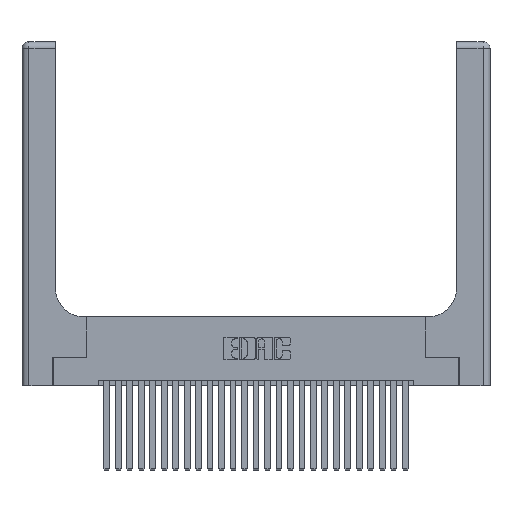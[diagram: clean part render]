
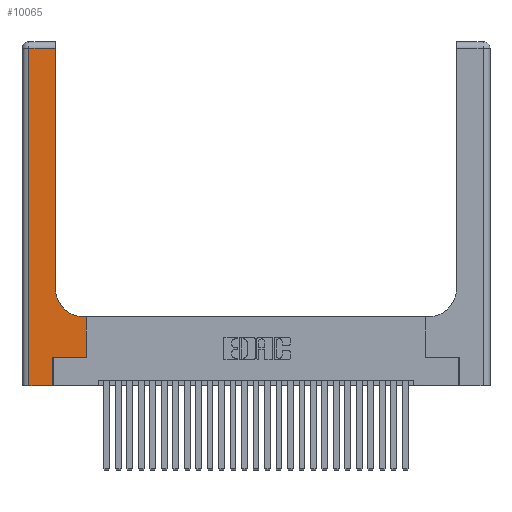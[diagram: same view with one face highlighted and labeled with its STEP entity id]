
A CAD part, top view. The second image highlights one B-rep face of the part: STEP entity #10065.
In plain terms, the highlighted planar face has unit normal (0, 0, 1).
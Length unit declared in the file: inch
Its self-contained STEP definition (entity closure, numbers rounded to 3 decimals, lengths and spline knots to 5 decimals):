
#229 = VERTEX_POINT ( 'NONE', #27348 ) ;
#466 = CARTESIAN_POINT ( 'NONE',  ( 0.269, 0., 0.37 ) ) ;
#570 = AXIS2_PLACEMENT_3D ( 'NONE', #19030, #5917, #21131 ) ;
#973 = LINE ( 'NONE', #18431, #23610 ) ;
#1056 = DIRECTION ( 'NONE',  ( 0., 1., 0. ) ) ;
#1150 = ORIENTED_EDGE ( 'NONE', *, *, #15504, .T. ) ;
#1578 = EDGE_CURVE ( 'NONE', #24084, #18993, #9985, .T. ) ;
#2184 = DIRECTION ( 'NONE',  ( 0., 0., -1. ) ) ;
#2525 = VERTEX_POINT ( 'NONE', #466 ) ;
#3880 = ORIENTED_EDGE ( 'NONE', *, *, #27745, .T. ) ;
#3969 = DIRECTION ( 'NONE',  ( 0., 1., 0. ) ) ;
#4430 = EDGE_CURVE ( 'NONE', #11971, #19254, #973, .T. ) ;
#4589 = VECTOR ( 'NONE', #25463, 39.37008 ) ;
#5917 = DIRECTION ( 'NONE',  ( 0., 0., -1. ) ) ;
#6012 = DIRECTION ( 'NONE',  ( 0., 1., 0. ) ) ;
#6155 = CARTESIAN_POINT ( 'NONE',  ( 0.5585, 0.25, 0.37 ) ) ;
#6886 = EDGE_LOOP ( 'NONE', ( #20039, #14225, #15555, #24863, #17990, #14328, #7619, #1150, #3880 ) ) ;
#7345 = VECTOR ( 'NONE', #1056, 39.37008 ) ;
#7619 = ORIENTED_EDGE ( 'NONE', *, *, #23731, .T. ) ;
#9127 = LINE ( 'NONE', #21754, #24862 ) ;
#9132 = LINE ( 'NONE', #6155, #25536 ) ;
#9709 = DIRECTION ( 'NONE',  ( 0., -1., 0. ) ) ;
#9985 = LINE ( 'NONE', #25466, #27654 ) ;
#10065 = ADVANCED_FACE ( 'NONE', ( #17483 ), #26066, .F. ) ;
#10351 = CARTESIAN_POINT ( 'NONE',  ( 0.5585, 0.6, 0.37 ) ) ;
#10888 = VECTOR ( 'NONE', #21321, 39.37008 ) ;
#11915 = CARTESIAN_POINT ( 'NONE',  ( 0.2915, 0.85, 0.37 ) ) ;
#11971 = VERTEX_POINT ( 'NONE', #19623 ) ;
#12785 = CARTESIAN_POINT ( 'NONE',  ( 0.5415, 0.6, 0.37 ) ) ;
#13074 = CARTESIAN_POINT ( 'NONE',  ( 0., 0., 0.37 ) ) ;
#13097 = VERTEX_POINT ( 'NONE', #12785 ) ;
#13257 = LINE ( 'NONE', #16658, #7345 ) ;
#14225 = ORIENTED_EDGE ( 'NONE', *, *, #16273, .T. ) ;
#14328 = ORIENTED_EDGE ( 'NONE', *, *, #27820, .T. ) ;
#14448 = VECTOR ( 'NONE', #17421, 39.37008 ) ;
#15504 = EDGE_CURVE ( 'NONE', #17314, #13097, #22275, .T. ) ;
#15509 = CARTESIAN_POINT ( 'NONE',  ( 0., 3., 0.37 ) ) ;
#15555 = ORIENTED_EDGE ( 'NONE', *, *, #4430, .T. ) ;
#16222 = VERTEX_POINT ( 'NONE', #17338 ) ;
#16273 = EDGE_CURVE ( 'NONE', #18993, #11971, #9127, .T. ) ;
#16658 = CARTESIAN_POINT ( 'NONE',  ( 0.269, 0., 0.37 ) ) ;
#17084 = CARTESIAN_POINT ( 'NONE',  ( 0.269, 0.25, 0.37 ) ) ;
#17314 = VERTEX_POINT ( 'NONE', #10351 ) ;
#17338 = CARTESIAN_POINT ( 'NONE',  ( 0.269, 0.25, 0.37 ) ) ;
#17421 = DIRECTION ( 'NONE',  ( 1., 0., 0. ) ) ;
#17483 = FACE_OUTER_BOUND ( 'NONE', #6886, .T. ) ;
#17701 = DIRECTION ( 'NONE',  ( -1., 0., 0. ) ) ;
#17990 = ORIENTED_EDGE ( 'NONE', *, *, #23566, .T. ) ;
#18431 = CARTESIAN_POINT ( 'NONE',  ( 0.06, 3., 0.37 ) ) ;
#18466 = CARTESIAN_POINT ( 'NONE',  ( 0.2915, 2.94, 0.37 ) ) ;
#18993 = VERTEX_POINT ( 'NONE', #18466 ) ;
#19030 = CARTESIAN_POINT ( 'NONE',  ( 0.5415, 0.85, 0.37 ) ) ;
#19223 = CARTESIAN_POINT ( 'NONE',  ( 0.2915, 0.6, 0.37 ) ) ;
#19254 = VERTEX_POINT ( 'NONE', #23219 ) ;
#19372 = EDGE_CURVE ( 'NONE', #19254, #2525, #20135, .T. ) ;
#19623 = CARTESIAN_POINT ( 'NONE',  ( 0.06, 2.94, 0.37 ) ) ;
#20039 = ORIENTED_EDGE ( 'NONE', *, *, #1578, .T. ) ;
#20135 = LINE ( 'NONE', #13074, #14448 ) ;
#20730 = AXIS2_PLACEMENT_3D ( 'NONE', #15509, #2184, #17701 ) ;
#21131 = DIRECTION ( 'NONE',  ( 1., 0., 0. ) ) ;
#21321 = DIRECTION ( 'NONE',  ( -1., 0., 0. ) ) ;
#21754 = CARTESIAN_POINT ( 'NONE',  ( 0., 2.94, 0.37 ) ) ;
#22275 = LINE ( 'NONE', #19223, #10888 ) ;
#23219 = CARTESIAN_POINT ( 'NONE',  ( 0.06, 0., 0.37 ) ) ;
#23290 = CIRCLE ( 'NONE', #570, 0.25 ) ;
#23566 = EDGE_CURVE ( 'NONE', #2525, #16222, #13257, .T. ) ;
#23610 = VECTOR ( 'NONE', #9709, 39.37008 ) ;
#23731 = EDGE_CURVE ( 'NONE', #229, #17314, #9132, .T. ) ;
#24084 = VERTEX_POINT ( 'NONE', #11915 ) ;
#24862 = VECTOR ( 'NONE', #25886, 39.37008 ) ;
#24863 = ORIENTED_EDGE ( 'NONE', *, *, #19372, .T. ) ;
#25463 = DIRECTION ( 'NONE',  ( 1., 0., 0. ) ) ;
#25466 = CARTESIAN_POINT ( 'NONE',  ( 0.2915, 3., 0.37 ) ) ;
#25536 = VECTOR ( 'NONE', #3969, 39.37008 ) ;
#25886 = DIRECTION ( 'NONE',  ( -1., 0., 0. ) ) ;
#26066 = PLANE ( 'NONE',  #20730 ) ;
#26900 = LINE ( 'NONE', #17084, #4589 ) ;
#27348 = CARTESIAN_POINT ( 'NONE',  ( 0.5585, 0.25, 0.37 ) ) ;
#27654 = VECTOR ( 'NONE', #6012, 39.37008 ) ;
#27745 = EDGE_CURVE ( 'NONE', #13097, #24084, #23290, .T. ) ;
#27820 = EDGE_CURVE ( 'NONE', #16222, #229, #26900, .T. ) ;
